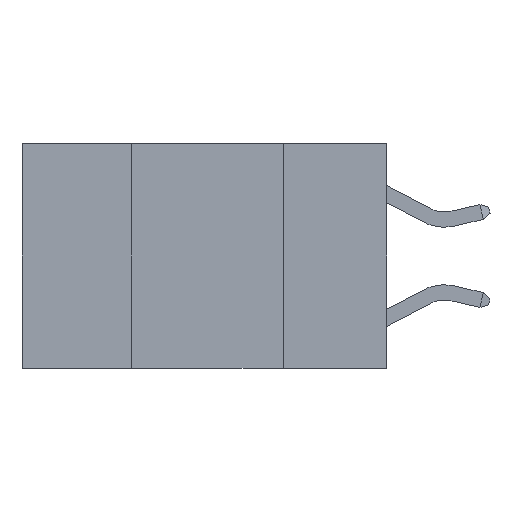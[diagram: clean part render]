
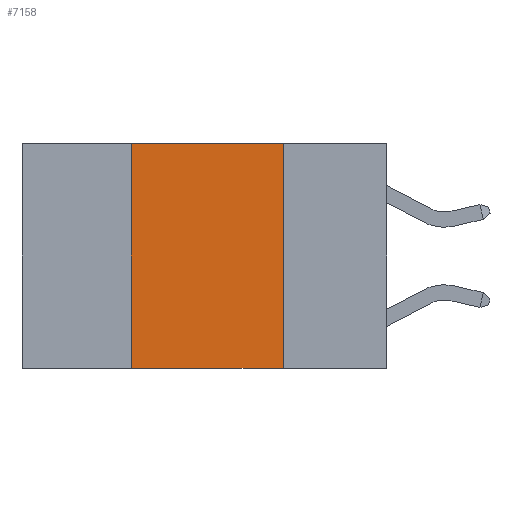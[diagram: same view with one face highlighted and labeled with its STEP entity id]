
A CAD part, left-side view. The second image highlights one B-rep face of the part: STEP entity #7158.
In plain terms, the highlighted planar face has unit normal (-1, 0, 0).
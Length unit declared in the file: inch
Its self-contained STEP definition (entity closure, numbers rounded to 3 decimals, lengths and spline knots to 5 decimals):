
#403 = VERTEX_POINT ( 'NONE', #1845 ) ;
#1592 = EDGE_LOOP ( 'NONE', ( #1720, #7344, #24596, #7933 ) ) ;
#1720 = ORIENTED_EDGE ( 'NONE', *, *, #21528, .F. ) ;
#1845 = CARTESIAN_POINT ( 'NONE',  ( 0., 0.42, -0.37 ) ) ;
#1858 = VECTOR ( 'NONE', #24577, 39.37008 ) ;
#1982 = VECTOR ( 'NONE', #17599, 39.37008 ) ;
#3341 = DIRECTION ( 'NONE',  ( 0., -1., 0. ) ) ;
#5307 = VECTOR ( 'NONE', #16356, 39.37008 ) ;
#5345 = PLANE ( 'NONE',  #26222 ) ;
#5768 = VERTEX_POINT ( 'NONE', #10473 ) ;
#5998 = CARTESIAN_POINT ( 'NONE',  ( 0., 0.6, 0. ) ) ;
#7158 = ADVANCED_FACE ( 'NONE', ( #26860 ), #5345, .F. ) ;
#7222 = VERTEX_POINT ( 'NONE', #22620 ) ;
#7344 = ORIENTED_EDGE ( 'NONE', *, *, #12372, .F. ) ;
#7834 = DIRECTION ( 'NONE',  ( 0., 0., -1. ) ) ;
#7933 = ORIENTED_EDGE ( 'NONE', *, *, #26890, .T. ) ;
#8861 = CARTESIAN_POINT ( 'NONE',  ( 0., 0.6, -0.37 ) ) ;
#10473 = CARTESIAN_POINT ( 'NONE',  ( 0., 0.17, 0. ) ) ;
#10816 = VECTOR ( 'NONE', #3341, 39.37008 ) ;
#12372 = EDGE_CURVE ( 'NONE', #7222, #5768, #15438, .T. ) ;
#13812 = VERTEX_POINT ( 'NONE', #23153 ) ;
#13843 = CARTESIAN_POINT ( 'NONE',  ( 0., 0.42, 0. ) ) ;
#14156 = LINE ( 'NONE', #13843, #5307 ) ;
#14919 = CARTESIAN_POINT ( 'NONE',  ( 0., 0.6, 0. ) ) ;
#15438 = LINE ( 'NONE', #5998, #1858 ) ;
#16356 = DIRECTION ( 'NONE',  ( 0., 0., 1. ) ) ;
#17599 = DIRECTION ( 'NONE',  ( 0., 0., -1. ) ) ;
#19789 = CARTESIAN_POINT ( 'NONE',  ( 0., 0.17, 0. ) ) ;
#21528 = EDGE_CURVE ( 'NONE', #5768, #13812, #22463, .T. ) ;
#22463 = LINE ( 'NONE', #19789, #1982 ) ;
#22547 = LINE ( 'NONE', #8861, #10816 ) ;
#22620 = CARTESIAN_POINT ( 'NONE',  ( 0., 0.42, 0. ) ) ;
#23153 = CARTESIAN_POINT ( 'NONE',  ( 0., 0.17, -0.37 ) ) ;
#24515 = DIRECTION ( 'NONE',  ( 1., 0., 0. ) ) ;
#24577 = DIRECTION ( 'NONE',  ( 0., -1., 0. ) ) ;
#24596 = ORIENTED_EDGE ( 'NONE', *, *, #28847, .F. ) ;
#26222 = AXIS2_PLACEMENT_3D ( 'NONE', #14919, #24515, #7834 ) ;
#26860 = FACE_OUTER_BOUND ( 'NONE', #1592, .T. ) ;
#26890 = EDGE_CURVE ( 'NONE', #403, #13812, #22547, .T. ) ;
#28847 = EDGE_CURVE ( 'NONE', #403, #7222, #14156, .T. ) ;
